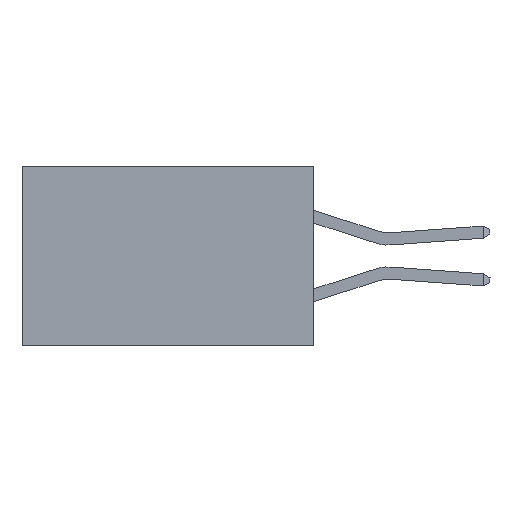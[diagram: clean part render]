
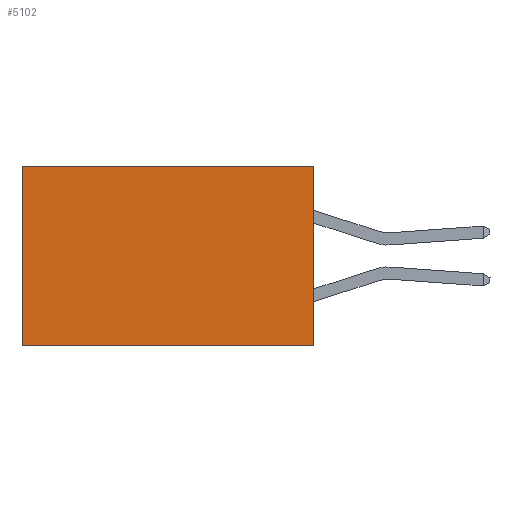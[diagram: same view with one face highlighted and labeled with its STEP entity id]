
A CAD part, left-side view. The second image highlights one B-rep face of the part: STEP entity #5102.
In plain terms, the highlighted planar face has unit normal (-1, 0, 0).
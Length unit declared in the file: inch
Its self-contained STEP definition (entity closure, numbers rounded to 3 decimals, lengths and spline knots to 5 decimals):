
#433 = CARTESIAN_POINT ( 'NONE',  ( 0.2875, 0.6, -0.37 ) ) ;
#513 = LINE ( 'NONE', #10469, #14798 ) ;
#608 = CARTESIAN_POINT ( 'NONE',  ( 0.2875, 0., 0. ) ) ;
#982 = CARTESIAN_POINT ( 'NONE',  ( 0.2875, 0., 0. ) ) ;
#1278 = CARTESIAN_POINT ( 'NONE',  ( 0.2875, 0., -0.37 ) ) ;
#2339 = ORIENTED_EDGE ( 'NONE', *, *, #16087, .F. ) ;
#3120 = DIRECTION ( 'NONE',  ( 0., 0., -1. ) ) ;
#3462 = VERTEX_POINT ( 'NONE', #433 ) ;
#3703 = VECTOR ( 'NONE', #3120, 39.37008 ) ;
#4522 = DIRECTION ( 'NONE',  ( 0., 0., -1. ) ) ;
#4989 = DIRECTION ( 'NONE',  ( 0., 0., -1. ) ) ;
#5102 = ADVANCED_FACE ( 'NONE', ( #18215 ), #7906, .F. ) ;
#5516 = DIRECTION ( 'NONE',  ( 0., 1., 0. ) ) ;
#6587 = EDGE_CURVE ( 'NONE', #17108, #16091, #10442, .T. ) ;
#7716 = CARTESIAN_POINT ( 'NONE',  ( 0.2875, 0.6, 0. ) ) ;
#7906 = PLANE ( 'NONE',  #18898 ) ;
#10442 = LINE ( 'NONE', #18757, #14782 ) ;
#10469 = CARTESIAN_POINT ( 'NONE',  ( 0.2875, 0., -0.37 ) ) ;
#10534 = DIRECTION ( 'NONE',  ( 0., 1., 0. ) ) ;
#10831 = LINE ( 'NONE', #982, #3703 ) ;
#12562 = ORIENTED_EDGE ( 'NONE', *, *, #20044, .T. ) ;
#13090 = EDGE_CURVE ( 'NONE', #17108, #14175, #10831, .T. ) ;
#13556 = CARTESIAN_POINT ( 'NONE',  ( 0.2875, 0.6, 0. ) ) ;
#14175 = VERTEX_POINT ( 'NONE', #1278 ) ;
#14782 = VECTOR ( 'NONE', #10534, 39.37008 ) ;
#14798 = VECTOR ( 'NONE', #5516, 39.37008 ) ;
#15095 = ORIENTED_EDGE ( 'NONE', *, *, #6587, .T. ) ;
#15447 = ORIENTED_EDGE ( 'NONE', *, *, #13090, .F. ) ;
#16087 = EDGE_CURVE ( 'NONE', #14175, #3462, #513, .T. ) ;
#16091 = VERTEX_POINT ( 'NONE', #13556 ) ;
#17108 = VERTEX_POINT ( 'NONE', #608 ) ;
#18022 = CARTESIAN_POINT ( 'NONE',  ( 0.2875, 0., 0. ) ) ;
#18213 = EDGE_LOOP ( 'NONE', ( #12562, #2339, #15447, #15095 ) ) ;
#18215 = FACE_OUTER_BOUND ( 'NONE', #18213, .T. ) ;
#18757 = CARTESIAN_POINT ( 'NONE',  ( 0.2875, 0., 0. ) ) ;
#18898 = AXIS2_PLACEMENT_3D ( 'NONE', #18022, #20901, #4989 ) ;
#19506 = VECTOR ( 'NONE', #4522, 39.37008 ) ;
#20044 = EDGE_CURVE ( 'NONE', #16091, #3462, #20514, .T. ) ;
#20514 = LINE ( 'NONE', #7716, #19506 ) ;
#20901 = DIRECTION ( 'NONE',  ( 1., 0., 0. ) ) ;
